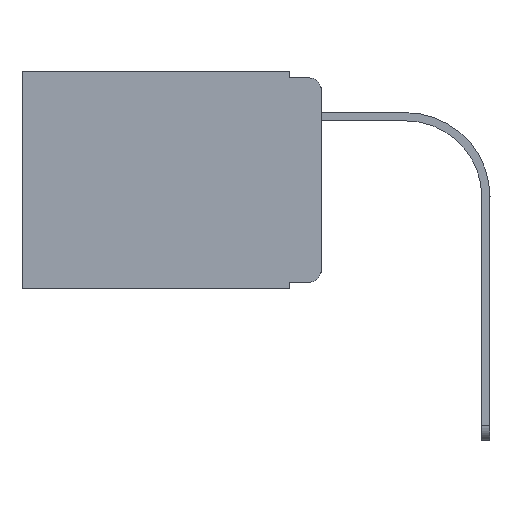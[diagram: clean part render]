
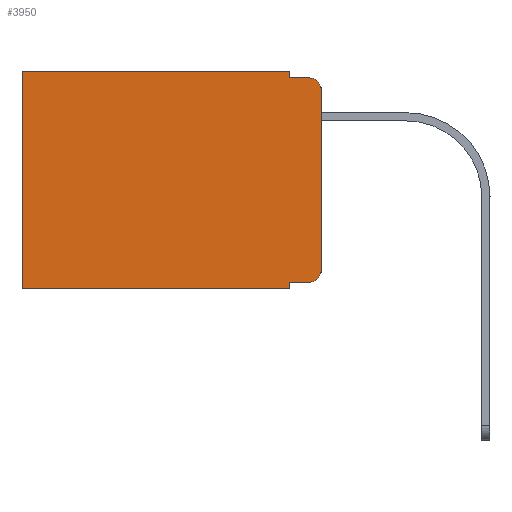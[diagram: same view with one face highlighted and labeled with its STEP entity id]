
A CAD part, left-side view. The second image highlights one B-rep face of the part: STEP entity #3950.
In plain terms, the highlighted planar face has unit normal (-1, 0, 0).
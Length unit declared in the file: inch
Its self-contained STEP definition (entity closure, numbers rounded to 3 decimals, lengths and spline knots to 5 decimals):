
#210 = LINE ( 'NONE', #6107, #5709 ) ;
#319 = AXIS2_PLACEMENT_3D ( 'NONE', #8690, #379, #3744 ) ;
#379 = DIRECTION ( 'NONE',  ( -1., 0., 0. ) ) ;
#483 = VERTEX_POINT ( 'NONE', #8888 ) ;
#565 = LINE ( 'NONE', #6450, #3521 ) ;
#594 = CARTESIAN_POINT ( 'NONE',  ( 0.298, 0.02, -0.03 ) ) ;
#726 = LINE ( 'NONE', #6713, #6069 ) ;
#927 = VERTEX_POINT ( 'NONE', #4587 ) ;
#962 = VERTEX_POINT ( 'NONE', #5364 ) ;
#1143 = ORIENTED_EDGE ( 'NONE', *, *, #3975, .F. ) ;
#1328 = VERTEX_POINT ( 'NONE', #6222 ) ;
#1553 = CARTESIAN_POINT ( 'NONE',  ( 0.298, 0., 0. ) ) ;
#1568 = VERTEX_POINT ( 'NONE', #10056 ) ;
#1656 = EDGE_CURVE ( 'NONE', #962, #1568, #7531, .T. ) ;
#1670 = CIRCLE ( 'NONE', #7279, 0.02 ) ;
#1673 = VECTOR ( 'NONE', #9952, 39.37008 ) ;
#1976 = CARTESIAN_POINT ( 'NONE',  ( 0.298, 0.473, 0. ) ) ;
#2049 = EDGE_CURVE ( 'NONE', #4930, #483, #10084, .T. ) ;
#2355 = EDGE_CURVE ( 'NONE', #483, #927, #565, .T. ) ;
#2682 = DIRECTION ( 'NONE',  ( 0., 1., 0. ) ) ;
#3154 = DIRECTION ( 'NONE',  ( 0., -1., 0. ) ) ;
#3185 = DIRECTION ( 'NONE',  ( 0., 0., -1. ) ) ;
#3214 = ORIENTED_EDGE ( 'NONE', *, *, #2049, .F. ) ;
#3284 = CARTESIAN_POINT ( 'NONE',  ( 0.298, 0.051, 0. ) ) ;
#3316 = VECTOR ( 'NONE', #7781, 39.37008 ) ;
#3521 = VECTOR ( 'NONE', #3154, 39.37008 ) ;
#3667 = ORIENTED_EDGE ( 'NONE', *, *, #9301, .T. ) ;
#3744 = DIRECTION ( 'NONE',  ( 0., 0., -1. ) ) ;
#3950 = ADVANCED_FACE ( 'NONE', ( #6075 ), #6547, .F. ) ;
#3963 = EDGE_CURVE ( 'NONE', #7677, #1328, #726, .T. ) ;
#3975 = EDGE_CURVE ( 'NONE', #9148, #6598, #10777, .T. ) ;
#4020 = ORIENTED_EDGE ( 'NONE', *, *, #3963, .F. ) ;
#4046 = LINE ( 'NONE', #8336, #4731 ) ;
#4282 = DIRECTION ( 'NONE',  ( 0., 0., -1. ) ) ;
#4587 = CARTESIAN_POINT ( 'NONE',  ( 0.298, 0.02, -0.01 ) ) ;
#4661 = AXIS2_PLACEMENT_3D ( 'NONE', #1553, #9892, #5069 ) ;
#4731 = VECTOR ( 'NONE', #6463, 39.37008 ) ;
#4869 = ORIENTED_EDGE ( 'NONE', *, *, #2355, .F. ) ;
#4876 = EDGE_CURVE ( 'NONE', #962, #7677, #4046, .T. ) ;
#4925 = VECTOR ( 'NONE', #2682, 39.37008 ) ;
#4930 = VERTEX_POINT ( 'NONE', #3284 ) ;
#4955 = CARTESIAN_POINT ( 'NONE',  ( 0.298, 0., -0.03 ) ) ;
#5069 = DIRECTION ( 'NONE',  ( 0., 0., -1. ) ) ;
#5199 = CARTESIAN_POINT ( 'NONE',  ( 0.298, 0.051, -0.343 ) ) ;
#5364 = CARTESIAN_POINT ( 'NONE',  ( 0.298, 0.051, -0.333 ) ) ;
#5709 = VECTOR ( 'NONE', #4282, 39.37008 ) ;
#5983 = CIRCLE ( 'NONE', #319, 0.02 ) ;
#6069 = VECTOR ( 'NONE', #7426, 39.37008 ) ;
#6075 = FACE_OUTER_BOUND ( 'NONE', #6602, .T. ) ;
#6107 = CARTESIAN_POINT ( 'NONE',  ( 0.298, 0.473, 0. ) ) ;
#6176 = EDGE_CURVE ( 'NONE', #4930, #9276, #10355, .T. ) ;
#6186 = CARTESIAN_POINT ( 'NONE',  ( 0.298, 0., 0. ) ) ;
#6222 = CARTESIAN_POINT ( 'NONE',  ( 0.298, 0.473, -0.343 ) ) ;
#6429 = DIRECTION ( 'NONE',  ( -1., 0., 0. ) ) ;
#6450 = CARTESIAN_POINT ( 'NONE',  ( 0.298, 0.051, -0.01 ) ) ;
#6463 = DIRECTION ( 'NONE',  ( 0., 0., -1. ) ) ;
#6547 = PLANE ( 'NONE',  #4661 ) ;
#6598 = VERTEX_POINT ( 'NONE', #7411 ) ;
#6602 = EDGE_LOOP ( 'NONE', ( #1143, #7564, #4869, #3214, #10307, #3667, #4020, #10497, #7720, #6643 ) ) ;
#6643 = ORIENTED_EDGE ( 'NONE', *, *, #8101, .T. ) ;
#6713 = CARTESIAN_POINT ( 'NONE',  ( 0.298, 0., -0.343 ) ) ;
#6770 = VECTOR ( 'NONE', #9235, 39.37008 ) ;
#7279 = AXIS2_PLACEMENT_3D ( 'NONE', #594, #6429, #3185 ) ;
#7411 = CARTESIAN_POINT ( 'NONE',  ( 0.298, 0., -0.313 ) ) ;
#7426 = DIRECTION ( 'NONE',  ( 0., 1., 0. ) ) ;
#7531 = LINE ( 'NONE', #10116, #6770 ) ;
#7564 = ORIENTED_EDGE ( 'NONE', *, *, #10498, .T. ) ;
#7677 = VERTEX_POINT ( 'NONE', #5199 ) ;
#7720 = ORIENTED_EDGE ( 'NONE', *, *, #1656, .T. ) ;
#7781 = DIRECTION ( 'NONE',  ( 0., 0., -1. ) ) ;
#8101 = EDGE_CURVE ( 'NONE', #1568, #6598, #5983, .T. ) ;
#8336 = CARTESIAN_POINT ( 'NONE',  ( 0.298, 0.051, 0. ) ) ;
#8439 = CARTESIAN_POINT ( 'NONE',  ( 0.298, 0.051, 0. ) ) ;
#8690 = CARTESIAN_POINT ( 'NONE',  ( 0.298, 0.02, -0.313 ) ) ;
#8888 = CARTESIAN_POINT ( 'NONE',  ( 0.298, 0.051, -0.01 ) ) ;
#9148 = VERTEX_POINT ( 'NONE', #4955 ) ;
#9235 = DIRECTION ( 'NONE',  ( 0., -1., 0. ) ) ;
#9276 = VERTEX_POINT ( 'NONE', #1976 ) ;
#9301 = EDGE_CURVE ( 'NONE', #9276, #1328, #210, .T. ) ;
#9892 = DIRECTION ( 'NONE',  ( 1., 0., 0. ) ) ;
#9952 = DIRECTION ( 'NONE',  ( 0., 0., -1. ) ) ;
#10056 = CARTESIAN_POINT ( 'NONE',  ( 0.298, 0.02, -0.333 ) ) ;
#10061 = CARTESIAN_POINT ( 'NONE',  ( 0.298, 0., 0. ) ) ;
#10084 = LINE ( 'NONE', #8439, #3316 ) ;
#10116 = CARTESIAN_POINT ( 'NONE',  ( 0.298, 0.051, -0.333 ) ) ;
#10307 = ORIENTED_EDGE ( 'NONE', *, *, #6176, .T. ) ;
#10355 = LINE ( 'NONE', #6186, #4925 ) ;
#10497 = ORIENTED_EDGE ( 'NONE', *, *, #4876, .F. ) ;
#10498 = EDGE_CURVE ( 'NONE', #9148, #927, #1670, .T. ) ;
#10777 = LINE ( 'NONE', #10061, #1673 ) ;
